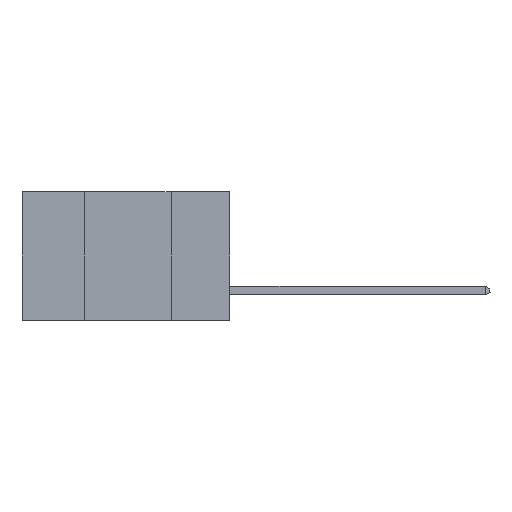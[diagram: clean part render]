
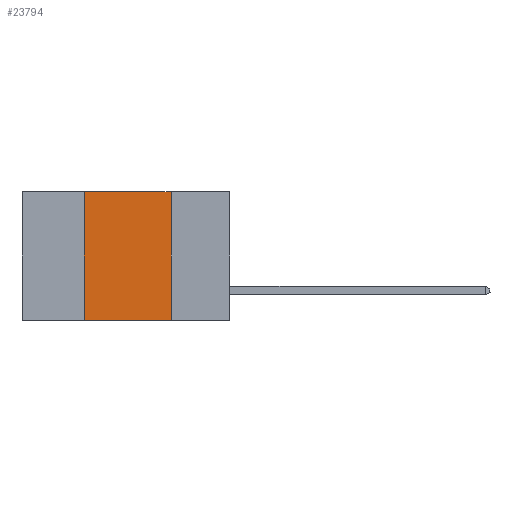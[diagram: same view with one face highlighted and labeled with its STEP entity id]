
A CAD part, left-side view. The second image highlights one B-rep face of the part: STEP entity #23794.
In plain terms, the highlighted planar face has unit normal (-1, 0, 0).
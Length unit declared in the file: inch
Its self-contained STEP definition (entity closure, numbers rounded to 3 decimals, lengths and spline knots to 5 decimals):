
#278 = DIRECTION ( 'NONE',  ( 0., -1., 0. ) ) ;
#499 = CARTESIAN_POINT ( 'NONE',  ( 0., 0.17, 0. ) ) ;
#1099 = LINE ( 'NONE', #4835, #24443 ) ;
#1126 = LINE ( 'NONE', #18096, #19881 ) ;
#1130 = VERTEX_POINT ( 'NONE', #499 ) ;
#1318 = LINE ( 'NONE', #28581, #25680 ) ;
#1820 = CARTESIAN_POINT ( 'NONE',  ( 0., 0.17, -0.37 ) ) ;
#2071 = AXIS2_PLACEMENT_3D ( 'NONE', #13887, #9039, #20480 ) ;
#3613 = VERTEX_POINT ( 'NONE', #19268 ) ;
#4641 = PLANE ( 'NONE',  #2071 ) ;
#4835 = CARTESIAN_POINT ( 'NONE',  ( 0., 0.17, 0. ) ) ;
#6269 = VECTOR ( 'NONE', #278, 39.37008 ) ;
#6410 = FACE_OUTER_BOUND ( 'NONE', #21240, .T. ) ;
#6926 = ORIENTED_EDGE ( 'NONE', *, *, #12870, .F. ) ;
#9039 = DIRECTION ( 'NONE',  ( 1., 0., 0. ) ) ;
#9825 = ORIENTED_EDGE ( 'NONE', *, *, #13509, .F. ) ;
#12316 = VERTEX_POINT ( 'NONE', #1820 ) ;
#12870 = EDGE_CURVE ( 'NONE', #3613, #1130, #1126, .T. ) ;
#13506 = CARTESIAN_POINT ( 'NONE',  ( 0., 0.6, -0.37 ) ) ;
#13509 = EDGE_CURVE ( 'NONE', #1130, #12316, #1099, .T. ) ;
#13887 = CARTESIAN_POINT ( 'NONE',  ( 0., 0.6, 0. ) ) ;
#16470 = EDGE_CURVE ( 'NONE', #28750, #3613, #1318, .T. ) ;
#17430 = ORIENTED_EDGE ( 'NONE', *, *, #25018, .T. ) ;
#18096 = CARTESIAN_POINT ( 'NONE',  ( 0., 0.6, 0. ) ) ;
#19268 = CARTESIAN_POINT ( 'NONE',  ( 0., 0.42, 0. ) ) ;
#19561 = DIRECTION ( 'NONE',  ( 0., 0., 1. ) ) ;
#19881 = VECTOR ( 'NONE', #22752, 39.37008 ) ;
#20480 = DIRECTION ( 'NONE',  ( 0., 0., -1. ) ) ;
#20581 = DIRECTION ( 'NONE',  ( 0., 0., -1. ) ) ;
#21240 = EDGE_LOOP ( 'NONE', ( #9825, #6926, #24755, #17430 ) ) ;
#22752 = DIRECTION ( 'NONE',  ( 0., -1., 0. ) ) ;
#23794 = ADVANCED_FACE ( 'NONE', ( #6410 ), #4641, .F. ) ;
#24443 = VECTOR ( 'NONE', #20581, 39.37008 ) ;
#24755 = ORIENTED_EDGE ( 'NONE', *, *, #16470, .F. ) ;
#25018 = EDGE_CURVE ( 'NONE', #28750, #12316, #27157, .T. ) ;
#25680 = VECTOR ( 'NONE', #19561, 39.37008 ) ;
#27157 = LINE ( 'NONE', #13506, #6269 ) ;
#28581 = CARTESIAN_POINT ( 'NONE',  ( 0., 0.42, 0. ) ) ;
#28750 = VERTEX_POINT ( 'NONE', #28829 ) ;
#28829 = CARTESIAN_POINT ( 'NONE',  ( 0., 0.42, -0.37 ) ) ;
